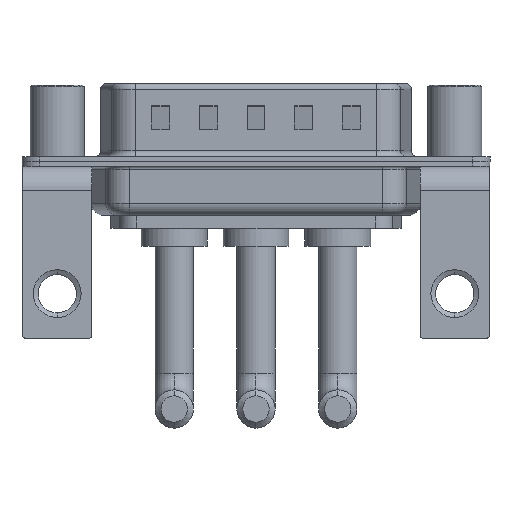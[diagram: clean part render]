
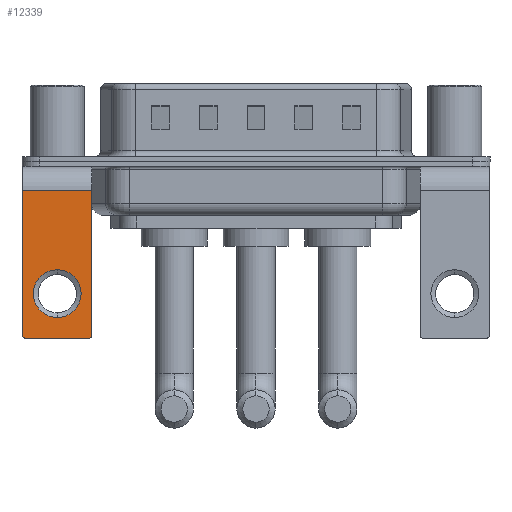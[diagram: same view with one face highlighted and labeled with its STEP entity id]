
A CAD part, front view. The second image highlights one B-rep face of the part: STEP entity #12339.
In plain terms, the highlighted planar face has unit normal (0, -1, 0).
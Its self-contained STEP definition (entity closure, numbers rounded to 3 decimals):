
#31 = VERTEX_POINT ( 'NONE', #12021 ) ;
#61 = CARTESIAN_POINT ( 'NONE',  ( 2.9, -6.25, -14.8 ) ) ;
#953 = ORIENTED_EDGE ( 'NONE', *, *, #5826, .T. ) ;
#1375 = DIRECTION ( 'NONE',  ( 0., 0., 1. ) ) ;
#1390 = CARTESIAN_POINT ( 'NONE',  ( -2.9, -6.25, -14.55 ) ) ;
#1817 = AXIS2_PLACEMENT_3D ( 'NONE', #2424, #8047, #9141 ) ;
#2301 = VERTEX_POINT ( 'NONE', #15598 ) ;
#2424 = CARTESIAN_POINT ( 'NONE',  ( 0., -6.25, -11.07 ) ) ;
#2896 = ORIENTED_EDGE ( 'NONE', *, *, #3598, .T. ) ;
#3406 = VERTEX_POINT ( 'NONE', #6715 ) ;
#3529 = CIRCLE ( 'NONE', #9107, 0.25 ) ;
#3596 = CARTESIAN_POINT ( 'NONE',  ( 0., -6.25, -11.07 ) ) ;
#3598 = EDGE_CURVE ( 'NONE', #17669, #2301, #3529, .T. ) ;
#3633 = VECTOR ( 'NONE', #11835, 1000. ) ;
#3851 = LINE ( 'NONE', #10574, #11865 ) ;
#4402 = DIRECTION ( 'NONE',  ( 0., 0., 1. ) ) ;
#4654 = LINE ( 'NONE', #6034, #3633 ) ;
#4711 = ORIENTED_EDGE ( 'NONE', *, *, #15505, .F. ) ;
#4876 = AXIS2_PLACEMENT_3D ( 'NONE', #14303, #8836, #8746 ) ;
#5179 = DIRECTION ( 'NONE',  ( 0., 0., 1. ) ) ;
#5447 = ORIENTED_EDGE ( 'NONE', *, *, #8870, .T. ) ;
#5771 = CARTESIAN_POINT ( 'NONE',  ( 2.9, -6.25, -2.4 ) ) ;
#5826 = EDGE_CURVE ( 'NONE', #7838, #6717, #10364, .T. ) ;
#6034 = CARTESIAN_POINT ( 'NONE',  ( 2.9, -6.25, -2.4 ) ) ;
#6134 = VERTEX_POINT ( 'NONE', #12623 ) ;
#6461 = ORIENTED_EDGE ( 'NONE', *, *, #15202, .T. ) ;
#6715 = CARTESIAN_POINT ( 'NONE',  ( 2.65, -6.25, -14.8 ) ) ;
#6717 = VERTEX_POINT ( 'NONE', #9973 ) ;
#6833 = ORIENTED_EDGE ( 'NONE', *, *, #9309, .F. ) ;
#7009 = AXIS2_PLACEMENT_3D ( 'NONE', #3596, #16303, #5179 ) ;
#7067 = LINE ( 'NONE', #5771, #11573 ) ;
#7838 = VERTEX_POINT ( 'NONE', #10768 ) ;
#8047 = DIRECTION ( 'NONE',  ( 0., 1., 0. ) ) ;
#8057 = CIRCLE ( 'NONE', #9232, 0.25 ) ;
#8272 = CARTESIAN_POINT ( 'NONE',  ( -2.65, -6.25, -14.55 ) ) ;
#8528 = EDGE_LOOP ( 'NONE', ( #953, #9264 ) ) ;
#8746 = DIRECTION ( 'NONE',  ( 0., 0., 1. ) ) ;
#8836 = DIRECTION ( 'NONE',  ( 0., 1., 0. ) ) ;
#8870 = EDGE_CURVE ( 'NONE', #3406, #31, #8057, .T. ) ;
#9107 = AXIS2_PLACEMENT_3D ( 'NONE', #8272, #11325, #4402 ) ;
#9141 = DIRECTION ( 'NONE',  ( 0., 0., 1. ) ) ;
#9232 = AXIS2_PLACEMENT_3D ( 'NONE', #18042, #11251, #1375 ) ;
#9264 = ORIENTED_EDGE ( 'NONE', *, *, #18060, .T. ) ;
#9309 = EDGE_CURVE ( 'NONE', #3406, #2301, #15533, .T. ) ;
#9973 = CARTESIAN_POINT ( 'NONE',  ( 0., -6.25, -9.07 ) ) ;
#10364 = CIRCLE ( 'NONE', #1817, 2. ) ;
#10574 = CARTESIAN_POINT ( 'NONE',  ( -2.9, -6.25, -2.4 ) ) ;
#10754 = VERTEX_POINT ( 'NONE', #11563 ) ;
#10768 = CARTESIAN_POINT ( 'NONE',  ( 0., -6.25, -13.07 ) ) ;
#11251 = DIRECTION ( 'NONE',  ( 0., -1., 0. ) ) ;
#11325 = DIRECTION ( 'NONE',  ( 0., -1., 0. ) ) ;
#11448 = FACE_BOUND ( 'NONE', #8528, .T. ) ;
#11563 = CARTESIAN_POINT ( 'NONE',  ( 2.9, -6.25, -2.4 ) ) ;
#11573 = VECTOR ( 'NONE', #15445, 1000. ) ;
#11835 = DIRECTION ( 'NONE',  ( 0., 0., -1. ) ) ;
#11865 = VECTOR ( 'NONE', #13707, 1000. ) ;
#12021 = CARTESIAN_POINT ( 'NONE',  ( 2.9, -6.25, -14.55 ) ) ;
#12339 = ADVANCED_FACE ( 'NONE', ( #11448, #17217 ), #13087, .F. ) ;
#12623 = CARTESIAN_POINT ( 'NONE',  ( -2.9, -6.25, -2.4 ) ) ;
#12878 = CIRCLE ( 'NONE', #7009, 2. ) ;
#13073 = VECTOR ( 'NONE', #16735, 1000. ) ;
#13087 = PLANE ( 'NONE',  #4876 ) ;
#13707 = DIRECTION ( 'NONE',  ( 0., 0., -1. ) ) ;
#14303 = CARTESIAN_POINT ( 'NONE',  ( 2.9, -6.25, -2.4 ) ) ;
#15202 = EDGE_CURVE ( 'NONE', #6134, #17669, #3851, .T. ) ;
#15379 = EDGE_CURVE ( 'NONE', #10754, #6134, #7067, .T. ) ;
#15445 = DIRECTION ( 'NONE',  ( -1., 0., 0. ) ) ;
#15505 = EDGE_CURVE ( 'NONE', #10754, #31, #4654, .T. ) ;
#15533 = LINE ( 'NONE', #61, #13073 ) ;
#15596 = EDGE_LOOP ( 'NONE', ( #6461, #2896, #6833, #5447, #4711, #17995 ) ) ;
#15598 = CARTESIAN_POINT ( 'NONE',  ( -2.65, -6.25, -14.8 ) ) ;
#16303 = DIRECTION ( 'NONE',  ( 0., 1., 0. ) ) ;
#16735 = DIRECTION ( 'NONE',  ( -1., 0., 0. ) ) ;
#17217 = FACE_OUTER_BOUND ( 'NONE', #15596, .T. ) ;
#17669 = VERTEX_POINT ( 'NONE', #1390 ) ;
#17995 = ORIENTED_EDGE ( 'NONE', *, *, #15379, .T. ) ;
#18042 = CARTESIAN_POINT ( 'NONE',  ( 2.65, -6.25, -14.55 ) ) ;
#18060 = EDGE_CURVE ( 'NONE', #6717, #7838, #12878, .T. ) ;
